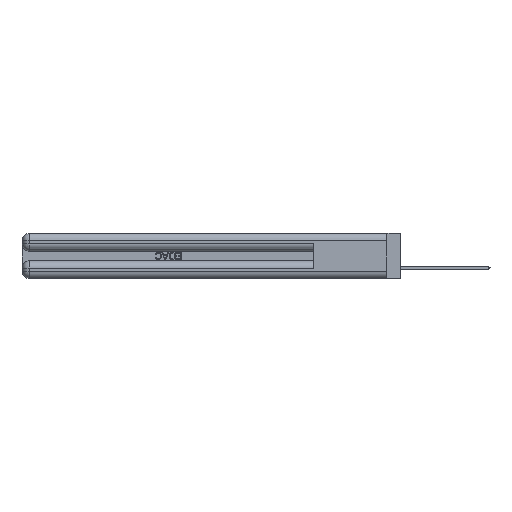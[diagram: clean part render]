
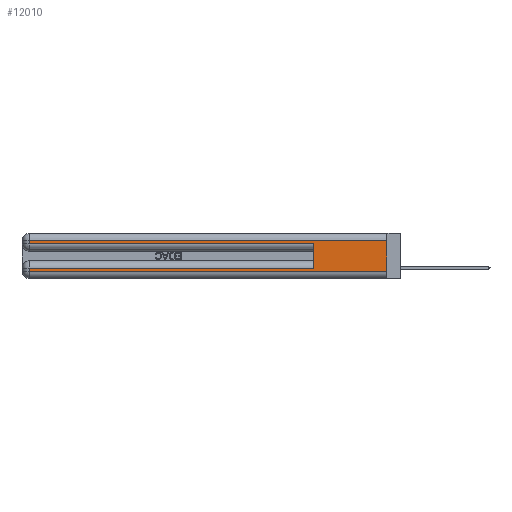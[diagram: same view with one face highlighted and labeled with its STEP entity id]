
A CAD part, left-side view. The second image highlights one B-rep face of the part: STEP entity #12010.
In plain terms, the highlighted planar face has unit normal (-1, 0, 0).
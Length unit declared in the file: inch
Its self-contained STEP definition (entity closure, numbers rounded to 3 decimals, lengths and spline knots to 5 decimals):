
#411 = VERTEX_POINT ( 'NONE', #28494 ) ;
#1352 = CARTESIAN_POINT ( 'NONE',  ( 0., 2.94, 0.37 ) ) ;
#1516 = VECTOR ( 'NONE', #14215, 39.37008 ) ;
#1689 = CARTESIAN_POINT ( 'NONE',  ( 0., 0., 0.06 ) ) ;
#2381 = LINE ( 'NONE', #40047, #9087 ) ;
#3657 = VERTEX_POINT ( 'NONE', #53438 ) ;
#3901 = VERTEX_POINT ( 'NONE', #40154 ) ;
#4257 = ORIENTED_EDGE ( 'NONE', *, *, #11942, .T. ) ;
#5175 = ORIENTED_EDGE ( 'NONE', *, *, #15966, .F. ) ;
#6077 = CARTESIAN_POINT ( 'NONE',  ( 0., 0.6, 0.085 ) ) ;
#7007 = EDGE_LOOP ( 'NONE', ( #14523, #16034, #38272, #52749, #5175, #4257, #38788, #22634 ) ) ;
#8117 = VERTEX_POINT ( 'NONE', #48812 ) ;
#8319 = LINE ( 'NONE', #34302, #45379 ) ;
#8431 = VERTEX_POINT ( 'NONE', #32607 ) ;
#9087 = VECTOR ( 'NONE', #14843, 39.37008 ) ;
#9334 = DIRECTION ( 'NONE',  ( 0., 0., 1. ) ) ;
#9840 = CARTESIAN_POINT ( 'NONE',  ( 0., 0., 0.085 ) ) ;
#10127 = LINE ( 'NONE', #53225, #49960 ) ;
#10253 = VECTOR ( 'NONE', #12168, 39.37008 ) ;
#11939 = VECTOR ( 'NONE', #9334, 39.37008 ) ;
#11942 = EDGE_CURVE ( 'NONE', #16189, #3901, #48059, .T. ) ;
#12010 = ADVANCED_FACE ( 'NONE', ( #52732 ), #54193, .F. ) ;
#12168 = DIRECTION ( 'NONE',  ( 0., -1., 0. ) ) ;
#13210 = EDGE_CURVE ( 'NONE', #411, #3657, #30881, .T. ) ;
#14215 = DIRECTION ( 'NONE',  ( 0., 0., -1. ) ) ;
#14523 = ORIENTED_EDGE ( 'NONE', *, *, #38960, .F. ) ;
#14843 = DIRECTION ( 'NONE',  ( 0., 0., -1. ) ) ;
#15966 = EDGE_CURVE ( 'NONE', #16189, #3657, #45021, .T. ) ;
#16034 = ORIENTED_EDGE ( 'NONE', *, *, #38520, .T. ) ;
#16189 = VERTEX_POINT ( 'NONE', #6077 ) ;
#17070 = CARTESIAN_POINT ( 'NONE',  ( 0., 0., 0.285 ) ) ;
#18088 = CARTESIAN_POINT ( 'NONE',  ( 0., 0., 0.06 ) ) ;
#20264 = VECTOR ( 'NONE', #21994, 39.37008 ) ;
#20505 = DIRECTION ( 'NONE',  ( 0., 0., -1. ) ) ;
#21994 = DIRECTION ( 'NONE',  ( 0., -1., 0. ) ) ;
#22634 = ORIENTED_EDGE ( 'NONE', *, *, #30920, .T. ) ;
#24258 = VERTEX_POINT ( 'NONE', #40611 ) ;
#26944 = DIRECTION ( 'NONE',  ( 0., 1., 0. ) ) ;
#27634 = VECTOR ( 'NONE', #31178, 39.37008 ) ;
#28130 = DIRECTION ( 'NONE',  ( 0., 0., -1. ) ) ;
#28494 = CARTESIAN_POINT ( 'NONE',  ( 0., 2.94, 0.285 ) ) ;
#28887 = CARTESIAN_POINT ( 'NONE',  ( 0., 0., 0.37 ) ) ;
#30443 = EDGE_CURVE ( 'NONE', #8431, #411, #40811, .T. ) ;
#30881 = LINE ( 'NONE', #17070, #10253 ) ;
#30920 = EDGE_CURVE ( 'NONE', #24258, #54294, #50670, .T. ) ;
#31178 = DIRECTION ( 'NONE',  ( 0., 1., 0. ) ) ;
#31726 = CARTESIAN_POINT ( 'NONE',  ( 0., 0.6, 0.145 ) ) ;
#32607 = CARTESIAN_POINT ( 'NONE',  ( 0., 2.94, 0.31 ) ) ;
#34302 = CARTESIAN_POINT ( 'NONE',  ( 0., 0., 0.31 ) ) ;
#37403 = DIRECTION ( 'NONE',  ( 1., 0., 0. ) ) ;
#38272 = ORIENTED_EDGE ( 'NONE', *, *, #30443, .T. ) ;
#38520 = EDGE_CURVE ( 'NONE', #8117, #8431, #8319, .T. ) ;
#38788 = ORIENTED_EDGE ( 'NONE', *, *, #43258, .T. ) ;
#38960 = EDGE_CURVE ( 'NONE', #8117, #54294, #10127, .T. ) ;
#40047 = CARTESIAN_POINT ( 'NONE',  ( 0., 2.94, 0.37 ) ) ;
#40154 = CARTESIAN_POINT ( 'NONE',  ( 0., 2.94, 0.085 ) ) ;
#40611 = CARTESIAN_POINT ( 'NONE',  ( 0., 2.94, 0.06 ) ) ;
#40811 = LINE ( 'NONE', #1352, #1516 ) ;
#43258 = EDGE_CURVE ( 'NONE', #3901, #24258, #2381, .T. ) ;
#43827 = AXIS2_PLACEMENT_3D ( 'NONE', #28887, #37403, #20505 ) ;
#45021 = LINE ( 'NONE', #31726, #11939 ) ;
#45379 = VECTOR ( 'NONE', #26944, 39.37008 ) ;
#48059 = LINE ( 'NONE', #9840, #27634 ) ;
#48812 = CARTESIAN_POINT ( 'NONE',  ( 0., 0., 0.31 ) ) ;
#49960 = VECTOR ( 'NONE', #28130, 39.37008 ) ;
#50670 = LINE ( 'NONE', #18088, #20264 ) ;
#52732 = FACE_OUTER_BOUND ( 'NONE', #7007, .T. ) ;
#52749 = ORIENTED_EDGE ( 'NONE', *, *, #13210, .T. ) ;
#53225 = CARTESIAN_POINT ( 'NONE',  ( 0., 0., 0.37 ) ) ;
#53438 = CARTESIAN_POINT ( 'NONE',  ( 0., 0.6, 0.285 ) ) ;
#54193 = PLANE ( 'NONE',  #43827 ) ;
#54294 = VERTEX_POINT ( 'NONE', #1689 ) ;
